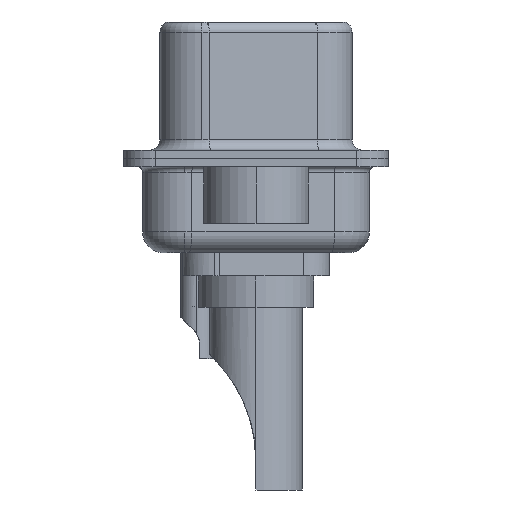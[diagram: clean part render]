
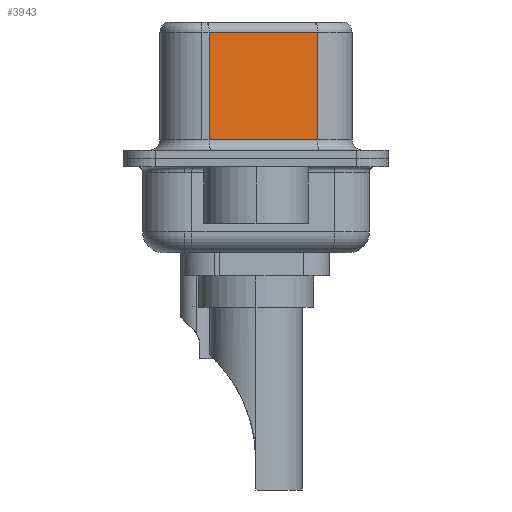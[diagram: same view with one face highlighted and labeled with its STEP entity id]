
A CAD part, left-side view. The second image highlights one B-rep face of the part: STEP entity #3943.
In plain terms, the highlighted planar face has unit normal (-0.985, -0.174, 0).
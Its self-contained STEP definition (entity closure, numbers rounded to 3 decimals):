
#1351 = VERTEX_POINT ( 'NONE', #3032 ) ;
#2303 = VERTEX_POINT ( 'NONE', #19015 ) ;
#3032 = CARTESIAN_POINT ( 'NONE',  ( 3.67, 2.233, 0.9 ) ) ;
#3943 = ADVANCED_FACE ( 'NONE', ( #5352 ), #10213, .F. ) ;
#5158 = CARTESIAN_POINT ( 'NONE',  ( 4.58, -2.927, 6.02 ) ) ;
#5352 = FACE_OUTER_BOUND ( 'NONE', #21639, .T. ) ;
#5436 = DIRECTION ( 'NONE',  ( -0.174, 0.985, 0. ) ) ;
#6211 = DIRECTION ( 'NONE',  ( 0.985, 0.174, 0. ) ) ;
#6801 = CARTESIAN_POINT ( 'NONE',  ( 4.58, -2.927, 6.02 ) ) ;
#7464 = LINE ( 'NONE', #11759, #12241 ) ;
#7500 = CARTESIAN_POINT ( 'NONE',  ( 4.58, -2.927, 6.52 ) ) ;
#8292 = DIRECTION ( 'NONE',  ( 0., 0., -1. ) ) ;
#8645 = DIRECTION ( 'NONE',  ( -0.174, 0.985, 0. ) ) ;
#8973 = LINE ( 'NONE', #19754, #17491 ) ;
#9416 = ORIENTED_EDGE ( 'NONE', *, *, #21644, .T. ) ;
#10213 = PLANE ( 'NONE',  #19113 ) ;
#10683 = VECTOR ( 'NONE', #8645, 1000. ) ;
#11311 = EDGE_CURVE ( 'NONE', #15423, #23322, #21850, .T. ) ;
#11759 = CARTESIAN_POINT ( 'NONE',  ( 4.58, -2.927, 0.9 ) ) ;
#12054 = CARTESIAN_POINT ( 'NONE',  ( 4.58, -2.927, 0.9 ) ) ;
#12144 = VECTOR ( 'NONE', #8292, 1000. ) ;
#12241 = VECTOR ( 'NONE', #22603, 1000. ) ;
#13938 = ORIENTED_EDGE ( 'NONE', *, *, #22485, .T. ) ;
#14879 = ORIENTED_EDGE ( 'NONE', *, *, #16513, .T. ) ;
#15423 = VERTEX_POINT ( 'NONE', #5158 ) ;
#16513 = EDGE_CURVE ( 'NONE', #1351, #23322, #7464, .T. ) ;
#17491 = VECTOR ( 'NONE', #23462, 1000. ) ;
#19015 = CARTESIAN_POINT ( 'NONE',  ( 3.67, 2.233, 6.02 ) ) ;
#19113 = AXIS2_PLACEMENT_3D ( 'NONE', #7500, #6211, #5436 ) ;
#19754 = CARTESIAN_POINT ( 'NONE',  ( 3.67, 2.233, 6.52 ) ) ;
#20345 = LINE ( 'NONE', #6801, #10683 ) ;
#20937 = CARTESIAN_POINT ( 'NONE',  ( 4.58, -2.927, 6.52 ) ) ;
#21639 = EDGE_LOOP ( 'NONE', ( #21834, #9416, #13938, #14879 ) ) ;
#21644 = EDGE_CURVE ( 'NONE', #15423, #2303, #20345, .T. ) ;
#21834 = ORIENTED_EDGE ( 'NONE', *, *, #11311, .F. ) ;
#21850 = LINE ( 'NONE', #20937, #12144 ) ;
#22485 = EDGE_CURVE ( 'NONE', #2303, #1351, #8973, .T. ) ;
#22603 = DIRECTION ( 'NONE',  ( 0.174, -0.985, 0. ) ) ;
#23322 = VERTEX_POINT ( 'NONE', #12054 ) ;
#23462 = DIRECTION ( 'NONE',  ( 0., 0., -1. ) ) ;
